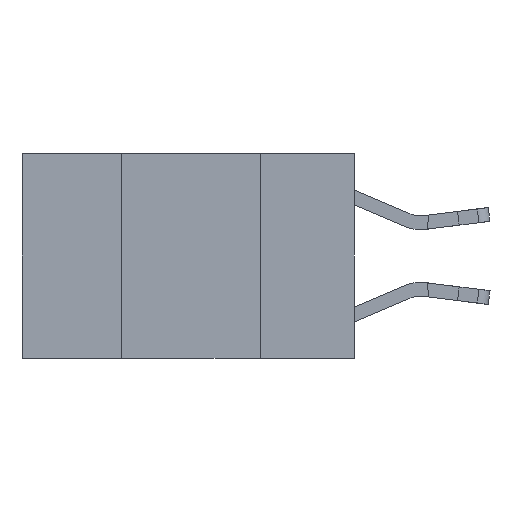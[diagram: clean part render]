
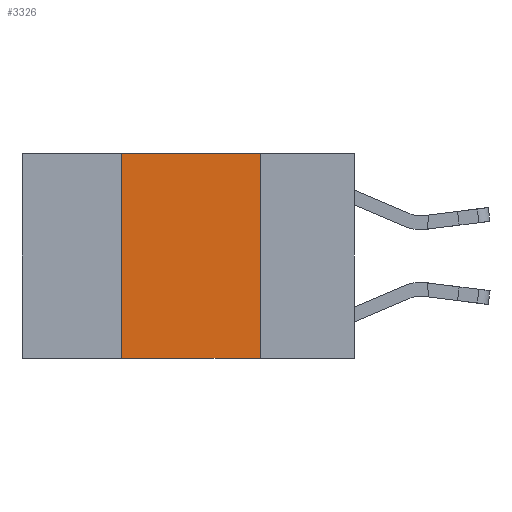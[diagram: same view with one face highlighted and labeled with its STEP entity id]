
A CAD part, left-side view. The second image highlights one B-rep face of the part: STEP entity #3326.
In plain terms, the highlighted planar face has unit normal (-1, 0, 0).
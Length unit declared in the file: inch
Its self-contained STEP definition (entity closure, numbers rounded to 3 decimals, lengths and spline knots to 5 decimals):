
#167 = VECTOR ( 'NONE', #8825, 39.37008 ) ;
#880 = DIRECTION ( 'NONE',  ( 0., -1., 0. ) ) ;
#1124 = CARTESIAN_POINT ( 'NONE',  ( 0., 0.42, -0.37 ) ) ;
#1167 = CARTESIAN_POINT ( 'NONE',  ( 0., 0.42, 0. ) ) ;
#1169 = VECTOR ( 'NONE', #880, 39.37008 ) ;
#1311 = VECTOR ( 'NONE', #4884, 39.37008 ) ;
#1482 = DIRECTION ( 'NONE',  ( 0., 0., -1. ) ) ;
#1932 = CARTESIAN_POINT ( 'NONE',  ( 0., 0.42, 0. ) ) ;
#2395 = LINE ( 'NONE', #5329, #8259 ) ;
#2742 = CARTESIAN_POINT ( 'NONE',  ( 0., 0.6, -0.37 ) ) ;
#3026 = EDGE_CURVE ( 'NONE', #6189, #3532, #9135, .T. ) ;
#3276 = VERTEX_POINT ( 'NONE', #4935 ) ;
#3326 = ADVANCED_FACE ( 'NONE', ( #8411 ), #4291, .F. ) ;
#3409 = AXIS2_PLACEMENT_3D ( 'NONE', #5464, #6444, #1482 ) ;
#3502 = DIRECTION ( 'NONE',  ( 0., -1., 0. ) ) ;
#3532 = VERTEX_POINT ( 'NONE', #1932 ) ;
#3834 = ORIENTED_EDGE ( 'NONE', *, *, #3026, .F. ) ;
#4291 = PLANE ( 'NONE',  #3409 ) ;
#4420 = EDGE_CURVE ( 'NONE', #6189, #6872, #10728, .T. ) ;
#4884 = DIRECTION ( 'NONE',  ( 0., 0., 1. ) ) ;
#4935 = CARTESIAN_POINT ( 'NONE',  ( 0., 0.17, 0. ) ) ;
#5329 = CARTESIAN_POINT ( 'NONE',  ( 0., 0.6, 0. ) ) ;
#5464 = CARTESIAN_POINT ( 'NONE',  ( 0., 0.6, 0. ) ) ;
#6189 = VERTEX_POINT ( 'NONE', #1124 ) ;
#6444 = DIRECTION ( 'NONE',  ( 1., 0., 0. ) ) ;
#6872 = VERTEX_POINT ( 'NONE', #12767 ) ;
#7137 = EDGE_CURVE ( 'NONE', #3532, #3276, #2395, .T. ) ;
#7594 = ORIENTED_EDGE ( 'NONE', *, *, #9735, .F. ) ;
#7926 = EDGE_LOOP ( 'NONE', ( #7594, #8802, #3834, #11958 ) ) ;
#8259 = VECTOR ( 'NONE', #3502, 39.37008 ) ;
#8411 = FACE_OUTER_BOUND ( 'NONE', #7926, .T. ) ;
#8802 = ORIENTED_EDGE ( 'NONE', *, *, #7137, .F. ) ;
#8825 = DIRECTION ( 'NONE',  ( 0., 0., -1. ) ) ;
#9135 = LINE ( 'NONE', #1167, #1311 ) ;
#9735 = EDGE_CURVE ( 'NONE', #3276, #6872, #12779, .T. ) ;
#9850 = CARTESIAN_POINT ( 'NONE',  ( 0., 0.17, 0. ) ) ;
#10728 = LINE ( 'NONE', #2742, #1169 ) ;
#11958 = ORIENTED_EDGE ( 'NONE', *, *, #4420, .T. ) ;
#12767 = CARTESIAN_POINT ( 'NONE',  ( 0., 0.17, -0.37 ) ) ;
#12779 = LINE ( 'NONE', #9850, #167 ) ;
